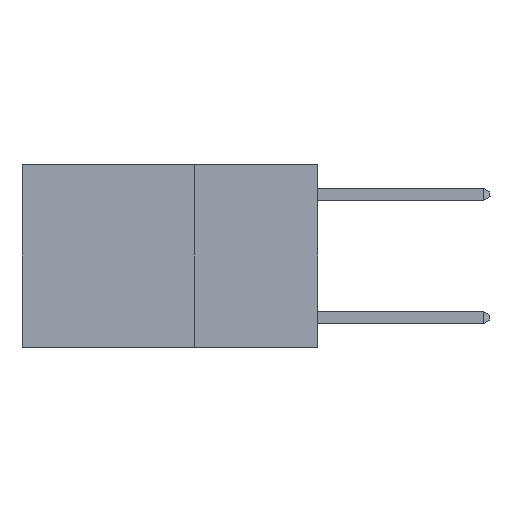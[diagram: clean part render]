
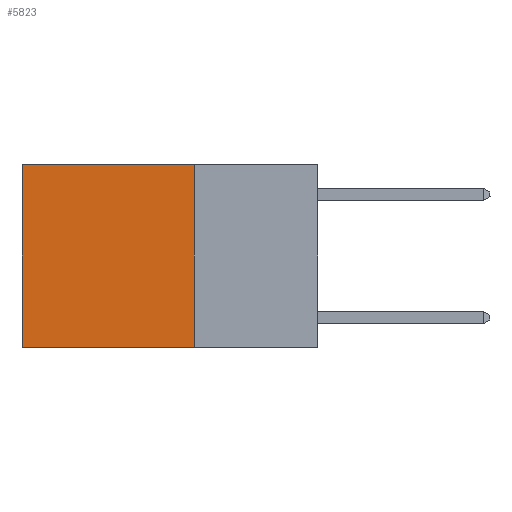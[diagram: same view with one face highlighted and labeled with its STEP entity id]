
A CAD part, left-side view. The second image highlights one B-rep face of the part: STEP entity #5823.
In plain terms, the highlighted planar face has unit normal (-1, 0, 0).
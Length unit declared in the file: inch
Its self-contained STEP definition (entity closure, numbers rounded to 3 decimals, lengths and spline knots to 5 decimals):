
#403 = LINE ( 'NONE', #17034, #19566 ) ;
#715 = ORIENTED_EDGE ( 'NONE', *, *, #11428, .T. ) ;
#1032 = VERTEX_POINT ( 'NONE', #8708 ) ;
#2669 = PLANE ( 'NONE',  #21597 ) ;
#4406 = EDGE_CURVE ( 'NONE', #11640, #1032, #24083, .T. ) ;
#4883 = ORIENTED_EDGE ( 'NONE', *, *, #5140, .T. ) ;
#4939 = CARTESIAN_POINT ( 'NONE',  ( 0.2625, 0.25, 0. ) ) ;
#5140 = EDGE_CURVE ( 'NONE', #11640, #14594, #6659, .T. ) ;
#5823 = ADVANCED_FACE ( 'NONE', ( #8285 ), #2669, .F. ) ;
#6049 = DIRECTION ( 'NONE',  ( 0., 0., -1. ) ) ;
#6659 = LINE ( 'NONE', #12880, #14671 ) ;
#7286 = DIRECTION ( 'NONE',  ( 0., 1., 0. ) ) ;
#7577 = CARTESIAN_POINT ( 'NONE',  ( 0.2625, 0.25, 0. ) ) ;
#8285 = FACE_OUTER_BOUND ( 'NONE', #17805, .T. ) ;
#8708 = CARTESIAN_POINT ( 'NONE',  ( 0.2625, 0.25, -0.37 ) ) ;
#8939 = VECTOR ( 'NONE', #18024, 39.37008 ) ;
#9638 = ORIENTED_EDGE ( 'NONE', *, *, #12841, .F. ) ;
#10220 = CARTESIAN_POINT ( 'NONE',  ( 0.2625, 0.6, 0. ) ) ;
#11038 = DIRECTION ( 'NONE',  ( 0., 0., -1. ) ) ;
#11428 = EDGE_CURVE ( 'NONE', #14594, #16756, #20475, .T. ) ;
#11640 = VERTEX_POINT ( 'NONE', #7577 ) ;
#11887 = CARTESIAN_POINT ( 'NONE',  ( 0.2625, 0.25, 0. ) ) ;
#12841 = EDGE_CURVE ( 'NONE', #1032, #16756, #403, .T. ) ;
#12880 = CARTESIAN_POINT ( 'NONE',  ( 0.2625, 0.25, 0. ) ) ;
#14594 = VERTEX_POINT ( 'NONE', #15793 ) ;
#14671 = VECTOR ( 'NONE', #18690, 39.37008 ) ;
#15774 = CARTESIAN_POINT ( 'NONE',  ( 0.2625, 0.6, -0.37 ) ) ;
#15793 = CARTESIAN_POINT ( 'NONE',  ( 0.2625, 0.6, 0. ) ) ;
#15871 = DIRECTION ( 'NONE',  ( 1., 0., 0. ) ) ;
#16756 = VERTEX_POINT ( 'NONE', #15774 ) ;
#17034 = CARTESIAN_POINT ( 'NONE',  ( 0.2625, 0.25, -0.37 ) ) ;
#17805 = EDGE_LOOP ( 'NONE', ( #715, #9638, #23328, #4883 ) ) ;
#18024 = DIRECTION ( 'NONE',  ( 0., 0., -1. ) ) ;
#18690 = DIRECTION ( 'NONE',  ( 0., 1., 0. ) ) ;
#19127 = VECTOR ( 'NONE', #11038, 39.37008 ) ;
#19566 = VECTOR ( 'NONE', #7286, 39.37008 ) ;
#20475 = LINE ( 'NONE', #10220, #8939 ) ;
#21597 = AXIS2_PLACEMENT_3D ( 'NONE', #11887, #15871, #6049 ) ;
#23328 = ORIENTED_EDGE ( 'NONE', *, *, #4406, .F. ) ;
#24083 = LINE ( 'NONE', #4939, #19127 ) ;
